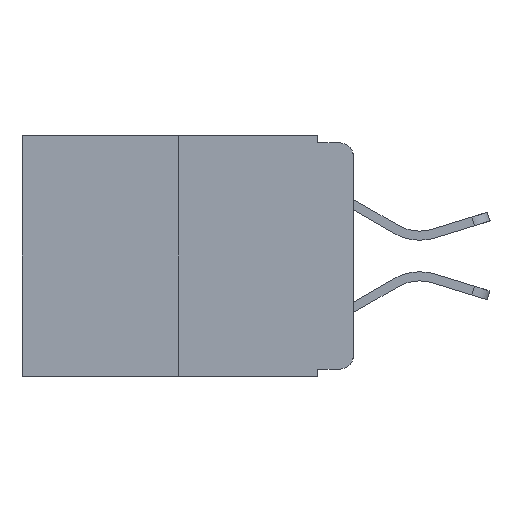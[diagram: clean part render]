
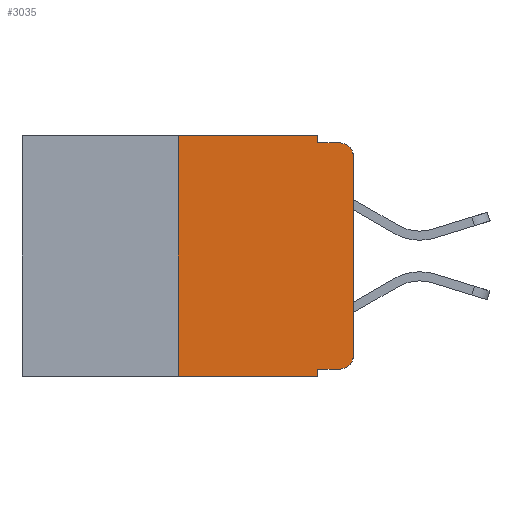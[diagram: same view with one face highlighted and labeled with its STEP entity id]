
A CAD part, left-side view. The second image highlights one B-rep face of the part: STEP entity #3035.
In plain terms, the highlighted planar face has unit normal (-1, 0, 0).
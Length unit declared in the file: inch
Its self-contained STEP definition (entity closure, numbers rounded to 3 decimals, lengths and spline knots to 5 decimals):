
#109 = EDGE_CURVE ( 'NONE', #4008, #4680, #13731, .T. ) ;
#283 = LINE ( 'NONE', #11957, #7119 ) ;
#390 = VECTOR ( 'NONE', #690, 39.37008 ) ;
#559 = CIRCLE ( 'NONE', #13107, 0.02 ) ;
#690 = DIRECTION ( 'NONE',  ( 0., 0., -1. ) ) ;
#843 = VERTEX_POINT ( 'NONE', #5569 ) ;
#1036 = EDGE_CURVE ( 'NONE', #4008, #13576, #13700, .T. ) ;
#1966 = EDGE_CURVE ( 'NONE', #16165, #843, #3085, .T. ) ;
#2202 = EDGE_CURVE ( 'NONE', #16165, #13576, #7332, .T. ) ;
#2224 = CARTESIAN_POINT ( 'NONE',  ( 0., 0., -0.313 ) ) ;
#2436 = EDGE_CURVE ( 'NONE', #843, #7186, #283, .T. ) ;
#2735 = DIRECTION ( 'NONE',  ( -1., 0., 0. ) ) ;
#2918 = CARTESIAN_POINT ( 'NONE',  ( 0., 0.02, -0.333 ) ) ;
#2952 = DIRECTION ( 'NONE',  ( -1., 0., 0. ) ) ;
#3018 = DIRECTION ( 'NONE',  ( 0., 0., -1. ) ) ;
#3035 = ADVANCED_FACE ( 'NONE', ( #8695 ), #4776, .F. ) ;
#3085 = LINE ( 'NONE', #10962, #16644 ) ;
#3148 = CARTESIAN_POINT ( 'NONE',  ( 0., 0.051, -0.01 ) ) ;
#3269 = VECTOR ( 'NONE', #11981, 39.37008 ) ;
#3284 = AXIS2_PLACEMENT_3D ( 'NONE', #15780, #7753, #3018 ) ;
#3372 = VECTOR ( 'NONE', #15260, 39.37008 ) ;
#3718 = VECTOR ( 'NONE', #6467, 39.37008 ) ;
#3780 = EDGE_CURVE ( 'NONE', #7186, #16818, #14538, .T. ) ;
#4008 = VERTEX_POINT ( 'NONE', #12413 ) ;
#4031 = CARTESIAN_POINT ( 'NONE',  ( 0., 0., 0. ) ) ;
#4680 = VERTEX_POINT ( 'NONE', #2918 ) ;
#4714 = EDGE_CURVE ( 'NONE', #16818, #15082, #6986, .T. ) ;
#4776 = PLANE ( 'NONE',  #3284 ) ;
#5569 = CARTESIAN_POINT ( 'NONE',  ( 0., 0.25, 0. ) ) ;
#5632 = EDGE_CURVE ( 'NONE', #8910, #15082, #559, .T. ) ;
#5868 = DIRECTION ( 'NONE',  ( 0., -1., 0. ) ) ;
#6467 = DIRECTION ( 'NONE',  ( 0., -1., 0. ) ) ;
#6986 = LINE ( 'NONE', #3148, #3372 ) ;
#7091 = ORIENTED_EDGE ( 'NONE', *, *, #1036, .F. ) ;
#7092 = AXIS2_PLACEMENT_3D ( 'NONE', #10766, #2735, #12069 ) ;
#7119 = VECTOR ( 'NONE', #5868, 39.37008 ) ;
#7186 = VERTEX_POINT ( 'NONE', #10239 ) ;
#7203 = VECTOR ( 'NONE', #8590, 39.37008 ) ;
#7237 = CARTESIAN_POINT ( 'NONE',  ( 0., 0., -0.03 ) ) ;
#7313 = CARTESIAN_POINT ( 'NONE',  ( 0., 0.25, -0.343 ) ) ;
#7332 = LINE ( 'NONE', #16115, #3718 ) ;
#7429 = EDGE_CURVE ( 'NONE', #9612, #8910, #13847, .T. ) ;
#7610 = CARTESIAN_POINT ( 'NONE',  ( 0., 0.051, -0.01 ) ) ;
#7749 = ORIENTED_EDGE ( 'NONE', *, *, #3780, .F. ) ;
#7753 = DIRECTION ( 'NONE',  ( 1., 0., 0. ) ) ;
#8590 = DIRECTION ( 'NONE',  ( 0., -1., 0. ) ) ;
#8636 = CARTESIAN_POINT ( 'NONE',  ( 0., 0.051, -0.343 ) ) ;
#8695 = FACE_OUTER_BOUND ( 'NONE', #16176, .T. ) ;
#8910 = VERTEX_POINT ( 'NONE', #7237 ) ;
#9370 = ORIENTED_EDGE ( 'NONE', *, *, #2202, .T. ) ;
#9612 = VERTEX_POINT ( 'NONE', #2224 ) ;
#10179 = CARTESIAN_POINT ( 'NONE',  ( 0., 0.051, -0.333 ) ) ;
#10196 = CARTESIAN_POINT ( 'NONE',  ( 0., 0.051, 0. ) ) ;
#10239 = CARTESIAN_POINT ( 'NONE',  ( 0., 0.051, 0. ) ) ;
#10267 = VECTOR ( 'NONE', #16751, 39.37008 ) ;
#10766 = CARTESIAN_POINT ( 'NONE',  ( 0., 0.02, -0.313 ) ) ;
#10962 = CARTESIAN_POINT ( 'NONE',  ( 0., 0.25, 0. ) ) ;
#10968 = CARTESIAN_POINT ( 'NONE',  ( 0., 0.02, -0.03 ) ) ;
#11957 = CARTESIAN_POINT ( 'NONE',  ( 0., 0.473, 0. ) ) ;
#11981 = DIRECTION ( 'NONE',  ( 0., 0., 1. ) ) ;
#12009 = ORIENTED_EDGE ( 'NONE', *, *, #1966, .F. ) ;
#12069 = DIRECTION ( 'NONE',  ( 0., 0., -1. ) ) ;
#12274 = DIRECTION ( 'NONE',  ( 0., 0., -1. ) ) ;
#12413 = CARTESIAN_POINT ( 'NONE',  ( 0., 0.051, -0.333 ) ) ;
#13107 = AXIS2_PLACEMENT_3D ( 'NONE', #10968, #2952, #12274 ) ;
#13355 = CARTESIAN_POINT ( 'NONE',  ( 0., 0.051, 0. ) ) ;
#13423 = ORIENTED_EDGE ( 'NONE', *, *, #7429, .T. ) ;
#13576 = VERTEX_POINT ( 'NONE', #8636 ) ;
#13700 = LINE ( 'NONE', #13355, #10267 ) ;
#13731 = LINE ( 'NONE', #10179, #7203 ) ;
#13847 = LINE ( 'NONE', #4031, #3269 ) ;
#14233 = ORIENTED_EDGE ( 'NONE', *, *, #4714, .F. ) ;
#14538 = LINE ( 'NONE', #10196, #390 ) ;
#14624 = ORIENTED_EDGE ( 'NONE', *, *, #2436, .F. ) ;
#14837 = ORIENTED_EDGE ( 'NONE', *, *, #109, .T. ) ;
#14899 = CIRCLE ( 'NONE', #7092, 0.02 ) ;
#15082 = VERTEX_POINT ( 'NONE', #16813 ) ;
#15260 = DIRECTION ( 'NONE',  ( 0., -1., 0. ) ) ;
#15780 = CARTESIAN_POINT ( 'NONE',  ( 0., 0.473, 0. ) ) ;
#16031 = ORIENTED_EDGE ( 'NONE', *, *, #16419, .T. ) ;
#16115 = CARTESIAN_POINT ( 'NONE',  ( 0., 0.473, -0.343 ) ) ;
#16165 = VERTEX_POINT ( 'NONE', #7313 ) ;
#16176 = EDGE_LOOP ( 'NONE', ( #13423, #16796, #14233, #7749, #14624, #12009, #9370, #7091, #14837, #16031 ) ) ;
#16419 = EDGE_CURVE ( 'NONE', #4680, #9612, #14899, .T. ) ;
#16644 = VECTOR ( 'NONE', #17120, 39.37008 ) ;
#16751 = DIRECTION ( 'NONE',  ( 0., 0., -1. ) ) ;
#16796 = ORIENTED_EDGE ( 'NONE', *, *, #5632, .T. ) ;
#16813 = CARTESIAN_POINT ( 'NONE',  ( 0., 0.02, -0.01 ) ) ;
#16818 = VERTEX_POINT ( 'NONE', #7610 ) ;
#17120 = DIRECTION ( 'NONE',  ( 0., 0., 1. ) ) ;
